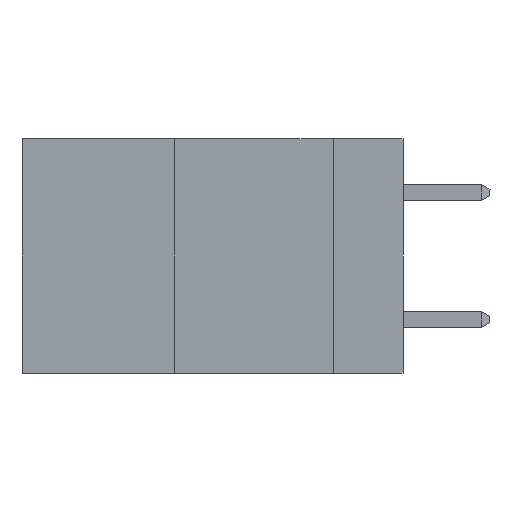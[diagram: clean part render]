
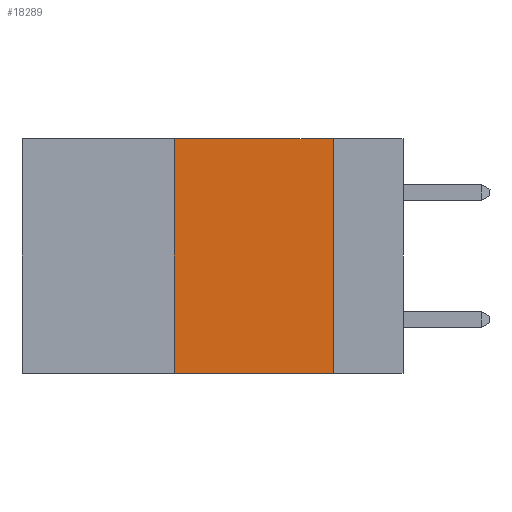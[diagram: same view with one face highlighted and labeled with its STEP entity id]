
A CAD part, left-side view. The second image highlights one B-rep face of the part: STEP entity #18289.
In plain terms, the highlighted planar face has unit normal (-1, 0, 0).
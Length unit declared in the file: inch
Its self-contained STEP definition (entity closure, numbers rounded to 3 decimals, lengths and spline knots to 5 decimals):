
#519 = DIRECTION ( 'NONE',  ( 0., 0., -1. ) ) ;
#719 = LINE ( 'NONE', #4054, #15847 ) ;
#1047 = FACE_OUTER_BOUND ( 'NONE', #6652, .T. ) ;
#1629 = LINE ( 'NONE', #11586, #9413 ) ;
#2596 = DIRECTION ( 'NONE',  ( 1., 0., 0. ) ) ;
#2820 = VERTEX_POINT ( 'NONE', #8235 ) ;
#3401 = CARTESIAN_POINT ( 'NONE',  ( 0., 0.11, 0. ) ) ;
#4054 = CARTESIAN_POINT ( 'NONE',  ( 0., 0.6, 0. ) ) ;
#4147 = CARTESIAN_POINT ( 'NONE',  ( 0., 0.36, -0.37 ) ) ;
#4604 = CARTESIAN_POINT ( 'NONE',  ( 0., 0.11, -0.37 ) ) ;
#4881 = EDGE_CURVE ( 'NONE', #8507, #18198, #14757, .T. ) ;
#6296 = LINE ( 'NONE', #3401, #13207 ) ;
#6502 = VECTOR ( 'NONE', #18005, 39.37008 ) ;
#6652 = EDGE_LOOP ( 'NONE', ( #16043, #16852, #17717, #18652 ) ) ;
#7405 = CARTESIAN_POINT ( 'NONE',  ( 0., 0.11, 0. ) ) ;
#8235 = CARTESIAN_POINT ( 'NONE',  ( 0., 0.36, 0. ) ) ;
#8507 = VERTEX_POINT ( 'NONE', #4147 ) ;
#9099 = EDGE_CURVE ( 'NONE', #2820, #12945, #719, .T. ) ;
#9413 = VECTOR ( 'NONE', #18634, 39.37008 ) ;
#9473 = EDGE_CURVE ( 'NONE', #8507, #2820, #1629, .T. ) ;
#11462 = PLANE ( 'NONE',  #15690 ) ;
#11586 = CARTESIAN_POINT ( 'NONE',  ( 0., 0.36, 0. ) ) ;
#12311 = CARTESIAN_POINT ( 'NONE',  ( 0., 0.6, -0.37 ) ) ;
#12945 = VERTEX_POINT ( 'NONE', #7405 ) ;
#12954 = DIRECTION ( 'NONE',  ( 0., 0., -1. ) ) ;
#13207 = VECTOR ( 'NONE', #519, 39.37008 ) ;
#14297 = CARTESIAN_POINT ( 'NONE',  ( 0., 0.6, 0. ) ) ;
#14439 = EDGE_CURVE ( 'NONE', #12945, #18198, #6296, .T. ) ;
#14757 = LINE ( 'NONE', #12311, #6502 ) ;
#15690 = AXIS2_PLACEMENT_3D ( 'NONE', #14297, #2596, #12954 ) ;
#15733 = DIRECTION ( 'NONE',  ( 0., -1., 0. ) ) ;
#15847 = VECTOR ( 'NONE', #15733, 39.37008 ) ;
#16043 = ORIENTED_EDGE ( 'NONE', *, *, #14439, .F. ) ;
#16852 = ORIENTED_EDGE ( 'NONE', *, *, #9099, .F. ) ;
#17717 = ORIENTED_EDGE ( 'NONE', *, *, #9473, .F. ) ;
#18005 = DIRECTION ( 'NONE',  ( 0., -1., 0. ) ) ;
#18198 = VERTEX_POINT ( 'NONE', #4604 ) ;
#18289 = ADVANCED_FACE ( 'NONE', ( #1047 ), #11462, .F. ) ;
#18634 = DIRECTION ( 'NONE',  ( 0., 0., 1. ) ) ;
#18652 = ORIENTED_EDGE ( 'NONE', *, *, #4881, .T. ) ;
